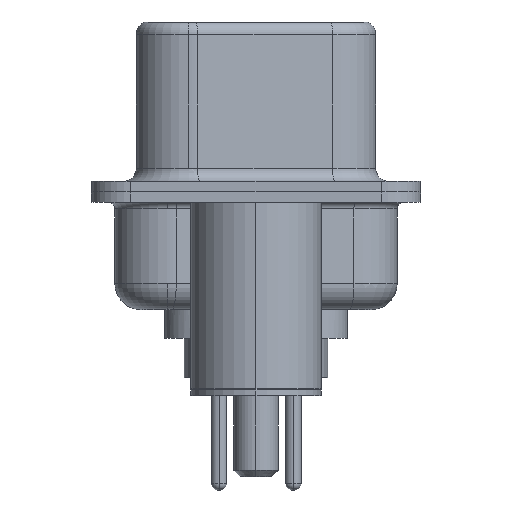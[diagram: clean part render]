
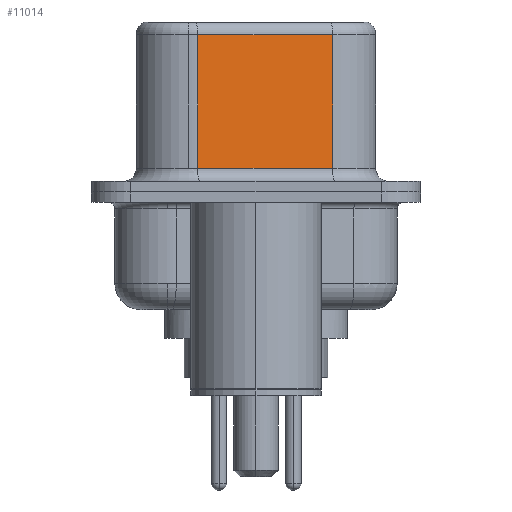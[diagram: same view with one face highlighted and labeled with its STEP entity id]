
A CAD part, left-side view. The second image highlights one B-rep face of the part: STEP entity #11014.
In plain terms, the highlighted planar face has unit normal (-0.985, -0.174, 0).
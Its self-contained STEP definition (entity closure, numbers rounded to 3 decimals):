
#611 = CARTESIAN_POINT ( 'NONE',  ( 4.565, -2.927, 6.52 ) ) ;
#683 = DIRECTION ( 'NONE',  ( 0., 0., -1. ) ) ;
#1033 = LINE ( 'NONE', #16912, #8859 ) ;
#1857 = LINE ( 'NONE', #611, #17590 ) ;
#2173 = VERTEX_POINT ( 'NONE', #3487 ) ;
#2354 = LINE ( 'NONE', #8137, #18122 ) ;
#2430 = DIRECTION ( 'NONE',  ( 0.985, 0.174, 0. ) ) ;
#3042 = CARTESIAN_POINT ( 'NONE',  ( 3.655, 2.233, 6.52 ) ) ;
#3487 = CARTESIAN_POINT ( 'NONE',  ( 4.565, -2.927, 6.02 ) ) ;
#4159 = CARTESIAN_POINT ( 'NONE',  ( 4.565, -2.927, 0.9 ) ) ;
#4599 = DIRECTION ( 'NONE',  ( 0., 0., -1. ) ) ;
#4606 = VERTEX_POINT ( 'NONE', #4159 ) ;
#6236 = CARTESIAN_POINT ( 'NONE',  ( 3.655, 2.233, 0.9 ) ) ;
#6330 = ORIENTED_EDGE ( 'NONE', *, *, #13768, .F. ) ;
#7728 = CARTESIAN_POINT ( 'NONE',  ( 3.655, 2.233, 6.02 ) ) ;
#8115 = AXIS2_PLACEMENT_3D ( 'NONE', #19193, #2430, #13199 ) ;
#8137 = CARTESIAN_POINT ( 'NONE',  ( 4.565, -2.927, 6.02 ) ) ;
#8859 = VECTOR ( 'NONE', #18517, 1000. ) ;
#9015 = LINE ( 'NONE', #3042, #16468 ) ;
#9430 = EDGE_CURVE ( 'NONE', #14379, #13910, #9015, .T. ) ;
#10759 = EDGE_CURVE ( 'NONE', #2173, #14379, #2354, .T. ) ;
#11014 = ADVANCED_FACE ( 'NONE', ( #15263 ), #11702, .F. ) ;
#11702 = PLANE ( 'NONE',  #8115 ) ;
#11895 = EDGE_LOOP ( 'NONE', ( #6330, #12491, #15842, #17981 ) ) ;
#12491 = ORIENTED_EDGE ( 'NONE', *, *, #10759, .T. ) ;
#13199 = DIRECTION ( 'NONE',  ( -0.174, 0.985, 0. ) ) ;
#13768 = EDGE_CURVE ( 'NONE', #2173, #4606, #1857, .T. ) ;
#13910 = VERTEX_POINT ( 'NONE', #6236 ) ;
#14379 = VERTEX_POINT ( 'NONE', #7728 ) ;
#15263 = FACE_OUTER_BOUND ( 'NONE', #11895, .T. ) ;
#15842 = ORIENTED_EDGE ( 'NONE', *, *, #9430, .T. ) ;
#16468 = VECTOR ( 'NONE', #4599, 1000. ) ;
#16912 = CARTESIAN_POINT ( 'NONE',  ( 4.565, -2.927, 0.9 ) ) ;
#17590 = VECTOR ( 'NONE', #683, 1000. ) ;
#17717 = EDGE_CURVE ( 'NONE', #13910, #4606, #1033, .T. ) ;
#17981 = ORIENTED_EDGE ( 'NONE', *, *, #17717, .T. ) ;
#18122 = VECTOR ( 'NONE', #18663, 1000. ) ;
#18517 = DIRECTION ( 'NONE',  ( 0.174, -0.985, 0. ) ) ;
#18663 = DIRECTION ( 'NONE',  ( -0.174, 0.985, 0. ) ) ;
#19193 = CARTESIAN_POINT ( 'NONE',  ( 4.565, -2.927, 6.52 ) ) ;
